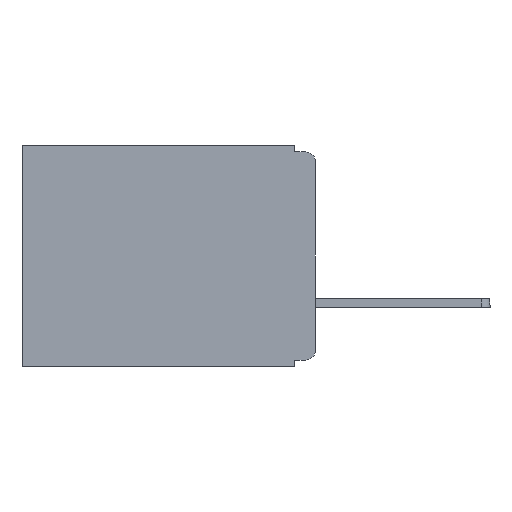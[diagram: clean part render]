
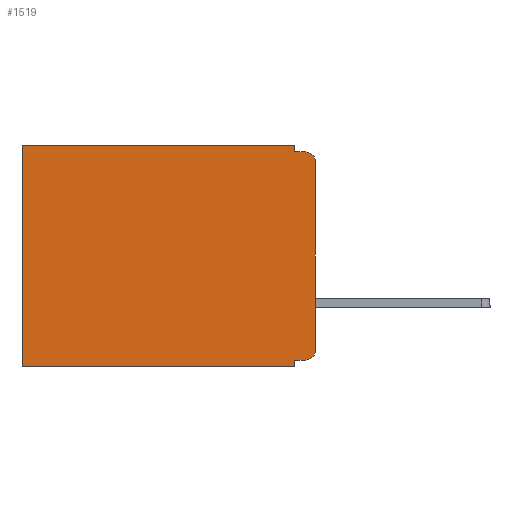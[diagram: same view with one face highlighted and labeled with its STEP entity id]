
A CAD part, left-side view. The second image highlights one B-rep face of the part: STEP entity #1519.
In plain terms, the highlighted planar face has unit normal (-1, 0, 0).
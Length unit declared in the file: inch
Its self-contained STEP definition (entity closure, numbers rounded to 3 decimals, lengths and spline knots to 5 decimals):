
#7 = CARTESIAN_POINT ( 'NONE',  ( 0.3, 0.015, -0.32 ) ) ;
#587 = DIRECTION ( 'NONE',  ( 0., 0., -1. ) ) ;
#703 = CIRCLE ( 'NONE', #3213, 0.015 ) ;
#728 = CARTESIAN_POINT ( 'NONE',  ( 0.3, 0., -0.33 ) ) ;
#765 = DIRECTION ( 'NONE',  ( 0., 0., -1. ) ) ;
#785 = DIRECTION ( 'NONE',  ( 1., 0., 0. ) ) ;
#929 = CARTESIAN_POINT ( 'NONE',  ( 0.3, 0., -0.32 ) ) ;
#1010 = DIRECTION ( 'NONE',  ( 0., 0., -1. ) ) ;
#1166 = VECTOR ( 'NONE', #3349, 39.37008 ) ;
#1172 = DIRECTION ( 'NONE',  ( -1., 0., 0. ) ) ;
#1194 = CARTESIAN_POINT ( 'NONE',  ( 0.3, 0.015, -0.025 ) ) ;
#1259 = ORIENTED_EDGE ( 'NONE', *, *, #5037, .F. ) ;
#1519 = ADVANCED_FACE ( 'NONE', ( #5125 ), #8470, .F. ) ;
#1811 = VERTEX_POINT ( 'NONE', #7 ) ;
#1964 = VERTEX_POINT ( 'NONE', #14623 ) ;
#2281 = DIRECTION ( 'NONE',  ( 0., 1., 0. ) ) ;
#2490 = LINE ( 'NONE', #8481, #12477 ) ;
#2996 = LINE ( 'NONE', #13613, #12172 ) ;
#3207 = DIRECTION ( 'NONE',  ( 0., 1., 0. ) ) ;
#3213 = AXIS2_PLACEMENT_3D ( 'NONE', #16331, #8661, #765 ) ;
#3349 = DIRECTION ( 'NONE',  ( 0., 0., -1. ) ) ;
#3473 = VERTEX_POINT ( 'NONE', #6688 ) ;
#3704 = VECTOR ( 'NONE', #2281, 39.37008 ) ;
#3855 = DIRECTION ( 'NONE',  ( 0., -1., 0. ) ) ;
#3959 = LINE ( 'NONE', #5628, #10919 ) ;
#4510 = EDGE_CURVE ( 'NONE', #6146, #6525, #7877, .T. ) ;
#4712 = LINE ( 'NONE', #11184, #1166 ) ;
#5037 = EDGE_CURVE ( 'NONE', #5623, #6525, #10508, .T. ) ;
#5125 = FACE_OUTER_BOUND ( 'NONE', #13751, .T. ) ;
#5203 = ORIENTED_EDGE ( 'NONE', *, *, #13502, .F. ) ;
#5263 = VERTEX_POINT ( 'NONE', #9254 ) ;
#5464 = VERTEX_POINT ( 'NONE', #10549 ) ;
#5623 = VERTEX_POINT ( 'NONE', #7057 ) ;
#5628 = CARTESIAN_POINT ( 'NONE',  ( 0.3, 0., -0.33 ) ) ;
#6146 = VERTEX_POINT ( 'NONE', #13062 ) ;
#6270 = CARTESIAN_POINT ( 'NONE',  ( 0.3, 0.015, -0.01 ) ) ;
#6476 = EDGE_CURVE ( 'NONE', #6146, #5464, #3959, .T. ) ;
#6525 = VERTEX_POINT ( 'NONE', #6270 ) ;
#6642 = CARTESIAN_POINT ( 'NONE',  ( 0.3, 0., 0. ) ) ;
#6688 = CARTESIAN_POINT ( 'NONE',  ( 0.3, 0.031, -0.32 ) ) ;
#7057 = CARTESIAN_POINT ( 'NONE',  ( 0.3, 0.031, -0.01 ) ) ;
#7193 = LINE ( 'NONE', #929, #3704 ) ;
#7451 = CARTESIAN_POINT ( 'NONE',  ( 0.3, 0.031, 0. ) ) ;
#7877 = CIRCLE ( 'NONE', #14288, 0.015 ) ;
#8136 = VERTEX_POINT ( 'NONE', #10720 ) ;
#8192 = VECTOR ( 'NONE', #16433, 39.37008 ) ;
#8470 = PLANE ( 'NONE',  #16081 ) ;
#8481 = CARTESIAN_POINT ( 'NONE',  ( 0.3, 0.437, -0.33 ) ) ;
#8661 = DIRECTION ( 'NONE',  ( -1., 0., 0. ) ) ;
#9254 = CARTESIAN_POINT ( 'NONE',  ( 0.3, 0.031, 0. ) ) ;
#9405 = VERTEX_POINT ( 'NONE', #10673 ) ;
#10205 = DIRECTION ( 'NONE',  ( 0., 0., -1. ) ) ;
#10293 = EDGE_CURVE ( 'NONE', #1964, #8136, #2490, .T. ) ;
#10508 = LINE ( 'NONE', #15242, #13139 ) ;
#10549 = CARTESIAN_POINT ( 'NONE',  ( 0.3, 0., -0.305 ) ) ;
#10626 = EDGE_CURVE ( 'NONE', #1811, #3473, #7193, .T. ) ;
#10673 = CARTESIAN_POINT ( 'NONE',  ( 0.3, 0.031, -0.33 ) ) ;
#10720 = CARTESIAN_POINT ( 'NONE',  ( 0.3, 0.437, -0.33 ) ) ;
#10846 = EDGE_CURVE ( 'NONE', #5263, #1964, #16796, .T. ) ;
#10919 = VECTOR ( 'NONE', #12342, 39.37008 ) ;
#10949 = ORIENTED_EDGE ( 'NONE', *, *, #6476, .F. ) ;
#11184 = CARTESIAN_POINT ( 'NONE',  ( 0.3, 0.031, -0.33 ) ) ;
#11345 = ORIENTED_EDGE ( 'NONE', *, *, #4510, .T. ) ;
#11656 = LINE ( 'NONE', #7451, #8192 ) ;
#11779 = EDGE_CURVE ( 'NONE', #3473, #9405, #4712, .T. ) ;
#12145 = ORIENTED_EDGE ( 'NONE', *, *, #10846, .T. ) ;
#12172 = VECTOR ( 'NONE', #3207, 39.37008 ) ;
#12342 = DIRECTION ( 'NONE',  ( 0., 0., -1. ) ) ;
#12477 = VECTOR ( 'NONE', #587, 39.37008 ) ;
#12529 = ORIENTED_EDGE ( 'NONE', *, *, #10293, .T. ) ;
#12939 = ORIENTED_EDGE ( 'NONE', *, *, #11779, .F. ) ;
#13062 = CARTESIAN_POINT ( 'NONE',  ( 0.3, 0., -0.025 ) ) ;
#13114 = DIRECTION ( 'NONE',  ( 0., 1., 0. ) ) ;
#13139 = VECTOR ( 'NONE', #3855, 39.37008 ) ;
#13502 = EDGE_CURVE ( 'NONE', #5263, #5623, #11656, .T. ) ;
#13613 = CARTESIAN_POINT ( 'NONE',  ( 0.3, 0., -0.33 ) ) ;
#13751 = EDGE_LOOP ( 'NONE', ( #10949, #11345, #1259, #5203, #12145, #12529, #15933, #12939, #16307, #16687 ) ) ;
#14288 = AXIS2_PLACEMENT_3D ( 'NONE', #1194, #1172, #1010 ) ;
#14623 = CARTESIAN_POINT ( 'NONE',  ( 0.3, 0.437, 0. ) ) ;
#15226 = EDGE_CURVE ( 'NONE', #1811, #5464, #703, .T. ) ;
#15242 = CARTESIAN_POINT ( 'NONE',  ( 0.3, 0., -0.01 ) ) ;
#15753 = EDGE_CURVE ( 'NONE', #9405, #8136, #2996, .T. ) ;
#15933 = ORIENTED_EDGE ( 'NONE', *, *, #15753, .F. ) ;
#16081 = AXIS2_PLACEMENT_3D ( 'NONE', #728, #785, #10205 ) ;
#16307 = ORIENTED_EDGE ( 'NONE', *, *, #10626, .F. ) ;
#16331 = CARTESIAN_POINT ( 'NONE',  ( 0.3, 0.015, -0.305 ) ) ;
#16419 = VECTOR ( 'NONE', #13114, 39.37008 ) ;
#16433 = DIRECTION ( 'NONE',  ( 0., 0., -1. ) ) ;
#16687 = ORIENTED_EDGE ( 'NONE', *, *, #15226, .T. ) ;
#16796 = LINE ( 'NONE', #6642, #16419 ) ;
